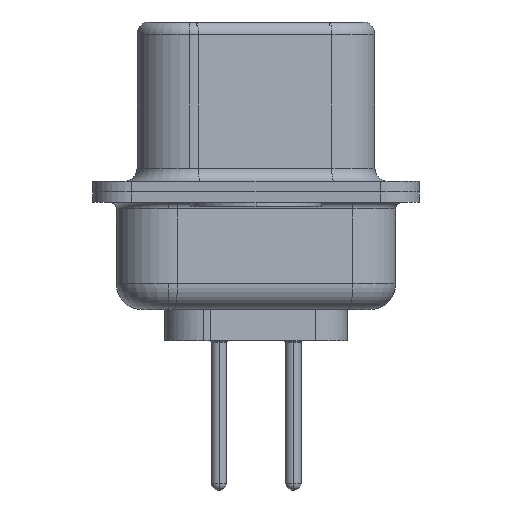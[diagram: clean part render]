
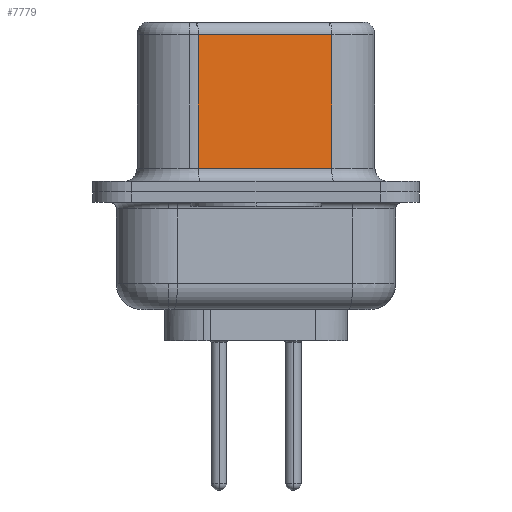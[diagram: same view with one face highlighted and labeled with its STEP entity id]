
A CAD part, left-side view. The second image highlights one B-rep face of the part: STEP entity #7779.
In plain terms, the highlighted planar face has unit normal (-0.985, -0.174, 0).
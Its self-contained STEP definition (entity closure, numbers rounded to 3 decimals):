
#325 = VECTOR ( 'NONE', #12191, 1000. ) ;
#778 = EDGE_CURVE ( 'NONE', #20956, #2709, #781, .T. ) ;
#781 = LINE ( 'NONE', #13214, #22792 ) ;
#1177 = LINE ( 'NONE', #11849, #325 ) ;
#1810 = LINE ( 'NONE', #9083, #20409 ) ;
#2139 = CARTESIAN_POINT ( 'NONE',  ( 3.68, 2.203, 6.02 ) ) ;
#2709 = VERTEX_POINT ( 'NONE', #2139 ) ;
#4191 = CARTESIAN_POINT ( 'NONE',  ( 4.58, -2.897, 6.02 ) ) ;
#4228 = CARTESIAN_POINT ( 'NONE',  ( 4.58, -2.897, 0.9 ) ) ;
#4375 = AXIS2_PLACEMENT_3D ( 'NONE', #20180, #14769, #21943 ) ;
#4909 = ORIENTED_EDGE ( 'NONE', *, *, #16363, .T. ) ;
#5210 = CARTESIAN_POINT ( 'NONE',  ( 3.68, 2.203, 0.9 ) ) ;
#5597 = VECTOR ( 'NONE', #21228, 1000. ) ;
#6912 = LINE ( 'NONE', #19464, #5597 ) ;
#7260 = VERTEX_POINT ( 'NONE', #4228 ) ;
#7779 = ADVANCED_FACE ( 'NONE', ( #14998 ), #16540, .F. ) ;
#8315 = ORIENTED_EDGE ( 'NONE', *, *, #778, .T. ) ;
#8673 = EDGE_CURVE ( 'NONE', #2709, #16369, #1177, .T. ) ;
#9083 = CARTESIAN_POINT ( 'NONE',  ( 4.58, -2.897, 0.9 ) ) ;
#9388 = EDGE_CURVE ( 'NONE', #20956, #7260, #6912, .T. ) ;
#11849 = CARTESIAN_POINT ( 'NONE',  ( 3.68, 2.203, 6.52 ) ) ;
#12191 = DIRECTION ( 'NONE',  ( 0., 0., -1. ) ) ;
#13214 = CARTESIAN_POINT ( 'NONE',  ( 4.58, -2.897, 6.02 ) ) ;
#14769 = DIRECTION ( 'NONE',  ( 0.985, 0.174, 0. ) ) ;
#14998 = FACE_OUTER_BOUND ( 'NONE', #23172, .T. ) ;
#15821 = ORIENTED_EDGE ( 'NONE', *, *, #8673, .T. ) ;
#16262 = DIRECTION ( 'NONE',  ( 0.174, -0.985, 0. ) ) ;
#16363 = EDGE_CURVE ( 'NONE', #16369, #7260, #1810, .T. ) ;
#16369 = VERTEX_POINT ( 'NONE', #5210 ) ;
#16540 = PLANE ( 'NONE',  #4375 ) ;
#17605 = ORIENTED_EDGE ( 'NONE', *, *, #9388, .F. ) ;
#19464 = CARTESIAN_POINT ( 'NONE',  ( 4.58, -2.897, 6.52 ) ) ;
#20180 = CARTESIAN_POINT ( 'NONE',  ( 4.58, -2.897, 6.52 ) ) ;
#20409 = VECTOR ( 'NONE', #16262, 1000. ) ;
#20838 = DIRECTION ( 'NONE',  ( -0.174, 0.985, 0. ) ) ;
#20956 = VERTEX_POINT ( 'NONE', #4191 ) ;
#21228 = DIRECTION ( 'NONE',  ( 0., 0., -1. ) ) ;
#21943 = DIRECTION ( 'NONE',  ( -0.174, 0.985, 0. ) ) ;
#22792 = VECTOR ( 'NONE', #20838, 1000. ) ;
#23172 = EDGE_LOOP ( 'NONE', ( #17605, #8315, #15821, #4909 ) ) ;
